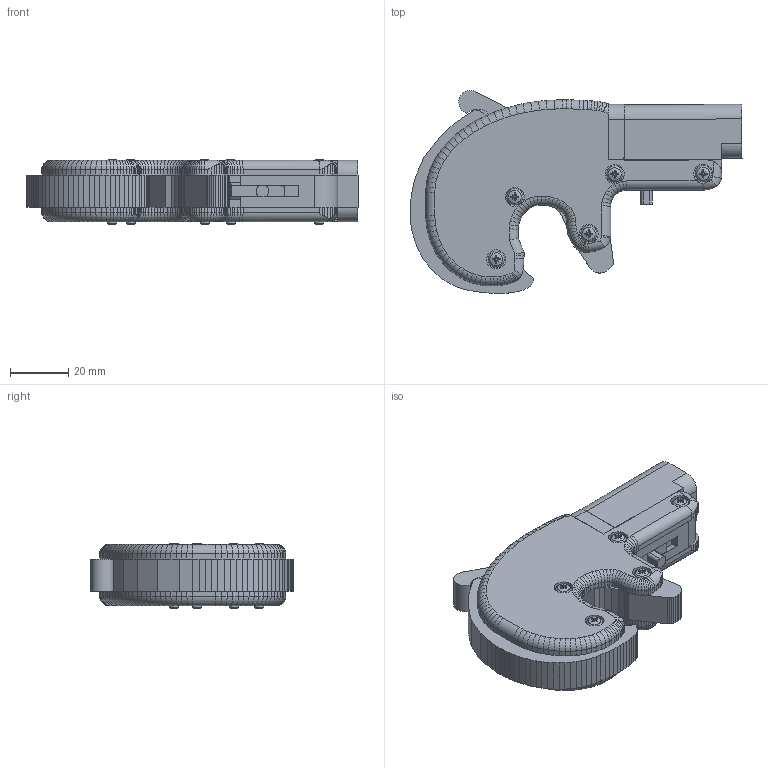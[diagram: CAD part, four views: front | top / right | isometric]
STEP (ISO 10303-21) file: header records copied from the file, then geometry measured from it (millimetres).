
FILE_DESCRIPTION((''),'2;1');
FILE_NAME('reprringer.stp','2013-07-11T16:55:12',('mrfr'),(''),'Autodesk Inventor 2013','Autodesk Inventor 2013','');
FILE_SCHEMA(('AUTOMOTIVE_DESIGN { 1 0 10303 214 1 1 1 1 }'));
Length unit declared in the file: millimetre
Products named in the file (16): Sestava; derringer_hlaven; derringer_mechanika; derringer_spoust; derringer_zapadka; derringer_zaver; derringer-LL; derringer-RR; Šroubový spoj; ISO 7045 Z M3 x 20 - 4.8 - Z; ISO 4035 M3; pruzina_mala
Assembly tree (23 placements, depth 3):
  Sestava
    derringer_hlaven
    derringer_mechanika
    derringer_spoust
    derringer_zapadka
    derringer_zaver
    derringer-LL
    derringer-RR
    Šroubový spoj
      ISO 7045 Z M3 x 20 - 4.8 - Z
      ISO 4035 M3
    Šroubový spoj
      ISO 7045 Z M3 x 20 - 4.8 - Z
      ISO 4035 M3
    Šroubový spoj
      ISO 7045 Z M3 x 20 - 4.8 - Z
      ISO 4035 M3
    Šroubový spoj
      ISO 7045 Z M3 x 20 - 4.8 - Z
      ISO 4035 M3
    Šroubový spoj
      ISO 7045 Z M3 x 20 - 4.8 - Z
      ISO 4035 M3
    pruzina_mala
Bounding box: 113.69 x 69.47 x 22.37 mm (x, y, z)
Volume: 75177.5 mm3; surface area: 36738.2 mm2
Topology: 18 solids, 18 shells, 1241 faces, 3255 edges, 2068 vertices
Faces by surface type: plane 789, cylinder 322, cone 100, torus 25, sphere 5
Full cylindrical faces by diameter (mm): 2 x1, 2.459 x5, 2.729 x5, 3 x19, 6 x1, 6.5 x5
Entity records: 31839 total; most frequent: CARTESIAN_POINT 6036, ORIENTED_EDGE 5332, DIRECTION 5136, EDGE_CURVE 2666, VECTOR 2154, LINE 2154, VERTEX_POINT 1704, AXIS2_PLACEMENT_3D 1491
